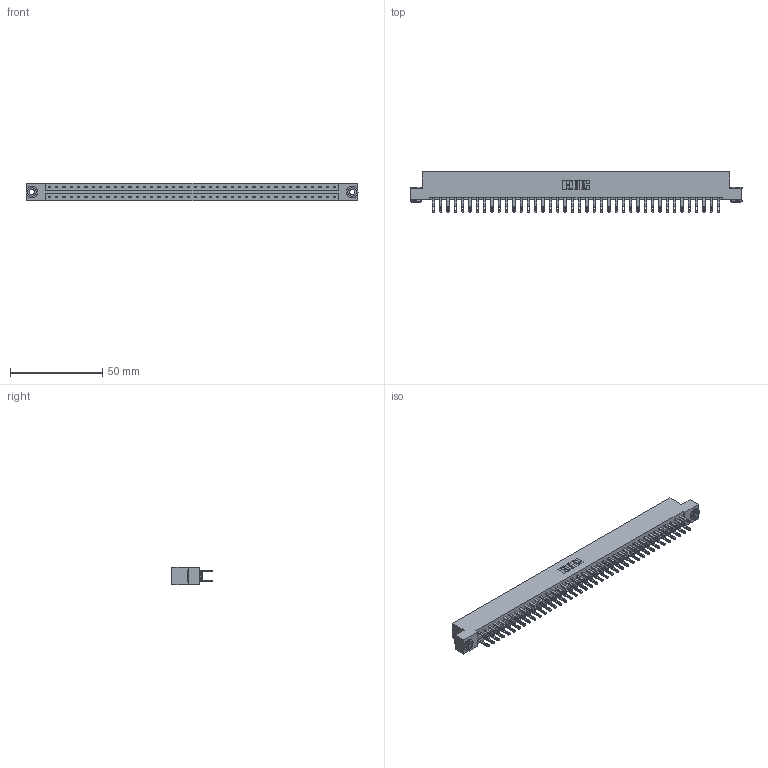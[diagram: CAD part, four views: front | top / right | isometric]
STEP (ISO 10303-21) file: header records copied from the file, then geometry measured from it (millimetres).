
FILE_DESCRIPTION (( 'STEP AP203' ), '1' );
FILE_NAME ('333-080-500-203.STEP', '2018-08-05T01:04:09', ( '' ), ( '' ), 'SwSTEP 2.0', 'SolidWorks 2016', '' );
FILE_SCHEMA (( 'CONFIG_CONTROL_DESIGN' ));
Length unit declared in the file: inch
Products named in the file (4): 333 Part_Flush - .156 Dia - TH; 345-292-001_345-293-100; 345-250-002_345-250-002-102; 333-080-500-203
Assembly tree (83 placements, depth 2):
  333-080-500-203
    333 Part_Flush - .156 Dia - TH
    345-292-001_345-293-100  x80
    345-250-002_345-250-002-102  x2
Bounding box: 180.04 x 21.85 x 9.4 mm (x, y, z)
Volume: 18625.7 mm3; surface area: 23100 mm2
Topology: 83 solids, 83 shells, 3992 faces, 12147 edges, 8094 vertices
Faces by surface type: plane 2480, cylinder 1504, cone 8
Entity records: 26572 total; most frequent: CARTESIAN_POINT 4381, ORIENTED_EDGE 4310, DIRECTION 3781, EDGE_CURVE 2155, LINE 1999, VECTOR 1999, VERTEX_POINT 1434, AXIS2_PLACEMENT_3D 891
